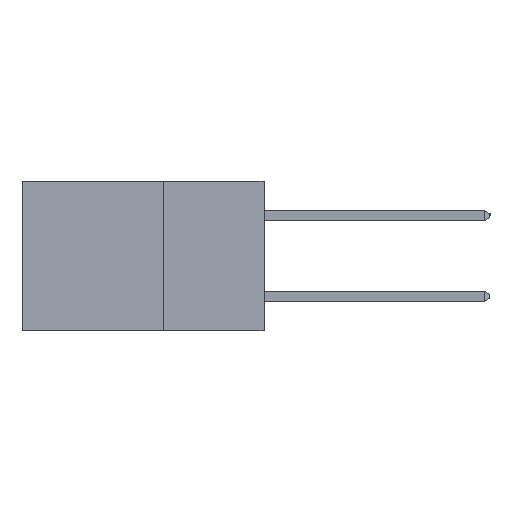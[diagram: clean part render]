
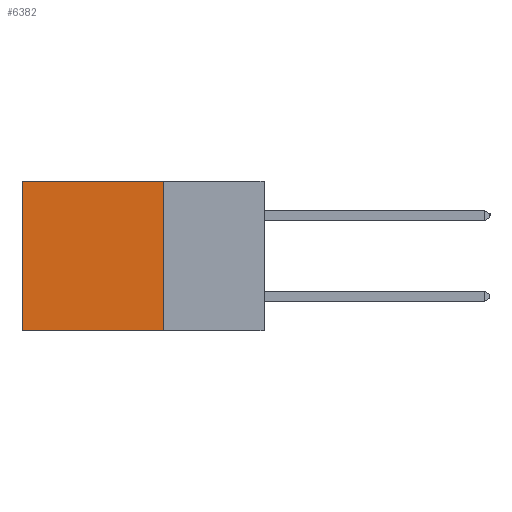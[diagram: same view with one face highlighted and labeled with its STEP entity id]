
A CAD part, left-side view. The second image highlights one B-rep face of the part: STEP entity #6382.
In plain terms, the highlighted planar face has unit normal (-1, 0, 0).
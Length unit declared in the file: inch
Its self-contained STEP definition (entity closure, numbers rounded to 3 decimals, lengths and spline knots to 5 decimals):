
#17 = ORIENTED_EDGE ( 'NONE', *, *, #192, .T. ) ;
#18 = VERTEX_POINT ( 'NONE', #1449 ) ;
#192 = EDGE_CURVE ( 'NONE', #18, #1303, #2673, .T. ) ;
#675 = EDGE_LOOP ( 'NONE', ( #17, #9671, #805, #3105 ) ) ;
#805 = ORIENTED_EDGE ( 'NONE', *, *, #11628, .F. ) ;
#1303 = VERTEX_POINT ( 'NONE', #12793 ) ;
#1359 = LINE ( 'NONE', #12511, #10034 ) ;
#1449 = CARTESIAN_POINT ( 'NONE',  ( 0.2615, 0.6, 0. ) ) ;
#1575 = CARTESIAN_POINT ( 'NONE',  ( 0.2615, 0.25, -0.37 ) ) ;
#1920 = AXIS2_PLACEMENT_3D ( 'NONE', #10912, #8758, #13150 ) ;
#2673 = LINE ( 'NONE', #9385, #5594 ) ;
#2967 = CARTESIAN_POINT ( 'NONE',  ( 0.2615, 0.25, -0.37 ) ) ;
#3105 = ORIENTED_EDGE ( 'NONE', *, *, #9191, .T. ) ;
#4118 = LINE ( 'NONE', #2967, #7693 ) ;
#4154 = CARTESIAN_POINT ( 'NONE',  ( 0.2615, 0.25, 0. ) ) ;
#4680 = CARTESIAN_POINT ( 'NONE',  ( 0.2615, 0.25, -0.37 ) ) ;
#4878 = DIRECTION ( 'NONE',  ( 0., 0., -1. ) ) ;
#5432 = PLANE ( 'NONE',  #1920 ) ;
#5437 = VERTEX_POINT ( 'NONE', #4680 ) ;
#5594 = VECTOR ( 'NONE', #10666, 39.37008 ) ;
#6111 = LINE ( 'NONE', #1575, #6586 ) ;
#6382 = ADVANCED_FACE ( 'NONE', ( #8977 ), #5432, .F. ) ;
#6586 = VECTOR ( 'NONE', #4878, 39.37008 ) ;
#7227 = EDGE_CURVE ( 'NONE', #5437, #1303, #4118, .T. ) ;
#7693 = VECTOR ( 'NONE', #9680, 39.37008 ) ;
#8038 = VERTEX_POINT ( 'NONE', #4154 ) ;
#8758 = DIRECTION ( 'NONE',  ( 1., 0., 0. ) ) ;
#8977 = FACE_OUTER_BOUND ( 'NONE', #675, .T. ) ;
#9191 = EDGE_CURVE ( 'NONE', #8038, #18, #1359, .T. ) ;
#9385 = CARTESIAN_POINT ( 'NONE',  ( 0.2615, 0.6, -0.37 ) ) ;
#9671 = ORIENTED_EDGE ( 'NONE', *, *, #7227, .F. ) ;
#9680 = DIRECTION ( 'NONE',  ( 0., 1., 0. ) ) ;
#10034 = VECTOR ( 'NONE', #13511, 39.37008 ) ;
#10666 = DIRECTION ( 'NONE',  ( 0., 0., -1. ) ) ;
#10912 = CARTESIAN_POINT ( 'NONE',  ( 0.2615, 0.25, -0.37 ) ) ;
#11628 = EDGE_CURVE ( 'NONE', #8038, #5437, #6111, .T. ) ;
#12511 = CARTESIAN_POINT ( 'NONE',  ( 0.2615, 0.25, 0. ) ) ;
#12793 = CARTESIAN_POINT ( 'NONE',  ( 0.2615, 0.6, -0.37 ) ) ;
#13150 = DIRECTION ( 'NONE',  ( 0., 0., -1. ) ) ;
#13511 = DIRECTION ( 'NONE',  ( 0., 1., 0. ) ) ;
